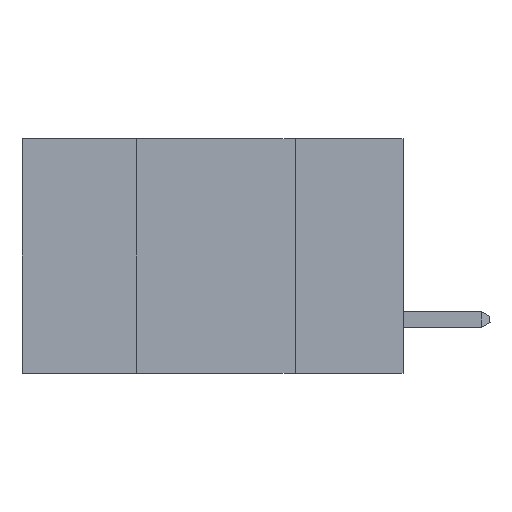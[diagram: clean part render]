
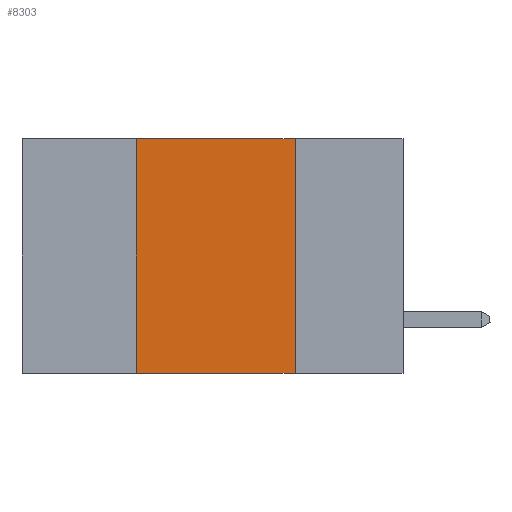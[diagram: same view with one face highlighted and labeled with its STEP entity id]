
A CAD part, left-side view. The second image highlights one B-rep face of the part: STEP entity #8303.
In plain terms, the highlighted planar face has unit normal (-1, 0, 0).
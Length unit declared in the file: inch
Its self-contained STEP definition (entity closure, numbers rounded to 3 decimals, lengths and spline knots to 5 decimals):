
#43 = EDGE_CURVE ( 'NONE', #9755, #3313, #2743, .T. ) ;
#287 = VECTOR ( 'NONE', #7212, 39.37008 ) ;
#1656 = LINE ( 'NONE', #8159, #287 ) ;
#2129 = DIRECTION ( 'NONE',  ( 0., 0., 1. ) ) ;
#2456 = PLANE ( 'NONE',  #4057 ) ;
#2743 = LINE ( 'NONE', #5092, #6846 ) ;
#3313 = VERTEX_POINT ( 'NONE', #9066 ) ;
#3629 = CARTESIAN_POINT ( 'NONE',  ( 0., 0.42, 0. ) ) ;
#3661 = DIRECTION ( 'NONE',  ( 0., 0., -1. ) ) ;
#3771 = ORIENTED_EDGE ( 'NONE', *, *, #5956, .F. ) ;
#4057 = AXIS2_PLACEMENT_3D ( 'NONE', #4114, #7363, #8951 ) ;
#4114 = CARTESIAN_POINT ( 'NONE',  ( 0., 0.6, 0. ) ) ;
#4430 = LINE ( 'NONE', #3629, #6101 ) ;
#4592 = CARTESIAN_POINT ( 'NONE',  ( 0., 0.42, -0.37 ) ) ;
#4858 = FACE_OUTER_BOUND ( 'NONE', #8438, .T. ) ;
#5092 = CARTESIAN_POINT ( 'NONE',  ( 0., 0.6, 0. ) ) ;
#5519 = LINE ( 'NONE', #10374, #7090 ) ;
#5897 = ORIENTED_EDGE ( 'NONE', *, *, #43, .F. ) ;
#5956 = EDGE_CURVE ( 'NONE', #3313, #7532, #5519, .T. ) ;
#5999 = DIRECTION ( 'NONE',  ( 0., -1., 0. ) ) ;
#6101 = VECTOR ( 'NONE', #2129, 39.37008 ) ;
#6294 = ORIENTED_EDGE ( 'NONE', *, *, #8546, .F. ) ;
#6645 = CARTESIAN_POINT ( 'NONE',  ( 0., 0.17, -0.37 ) ) ;
#6846 = VECTOR ( 'NONE', #5999, 39.37008 ) ;
#6906 = VERTEX_POINT ( 'NONE', #4592 ) ;
#7090 = VECTOR ( 'NONE', #3661, 39.37008 ) ;
#7212 = DIRECTION ( 'NONE',  ( 0., -1., 0. ) ) ;
#7363 = DIRECTION ( 'NONE',  ( 1., 0., 0. ) ) ;
#7532 = VERTEX_POINT ( 'NONE', #6645 ) ;
#8159 = CARTESIAN_POINT ( 'NONE',  ( 0., 0.6, -0.37 ) ) ;
#8303 = ADVANCED_FACE ( 'NONE', ( #4858 ), #2456, .F. ) ;
#8325 = EDGE_CURVE ( 'NONE', #6906, #7532, #1656, .T. ) ;
#8438 = EDGE_LOOP ( 'NONE', ( #3771, #5897, #6294, #8596 ) ) ;
#8546 = EDGE_CURVE ( 'NONE', #6906, #9755, #4430, .T. ) ;
#8596 = ORIENTED_EDGE ( 'NONE', *, *, #8325, .T. ) ;
#8951 = DIRECTION ( 'NONE',  ( 0., 0., -1. ) ) ;
#9041 = CARTESIAN_POINT ( 'NONE',  ( 0., 0.42, 0. ) ) ;
#9066 = CARTESIAN_POINT ( 'NONE',  ( 0., 0.17, 0. ) ) ;
#9755 = VERTEX_POINT ( 'NONE', #9041 ) ;
#10374 = CARTESIAN_POINT ( 'NONE',  ( 0., 0.17, 0. ) ) ;
